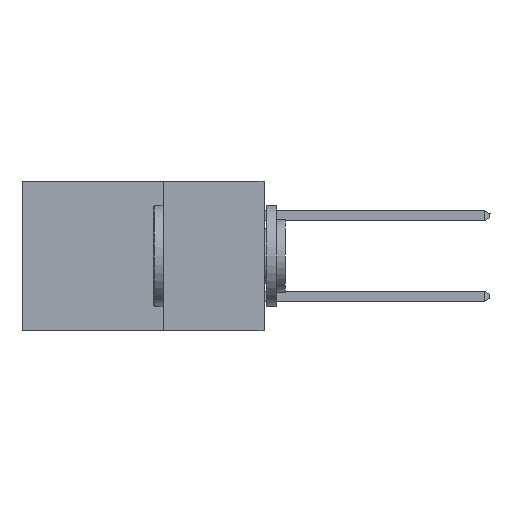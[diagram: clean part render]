
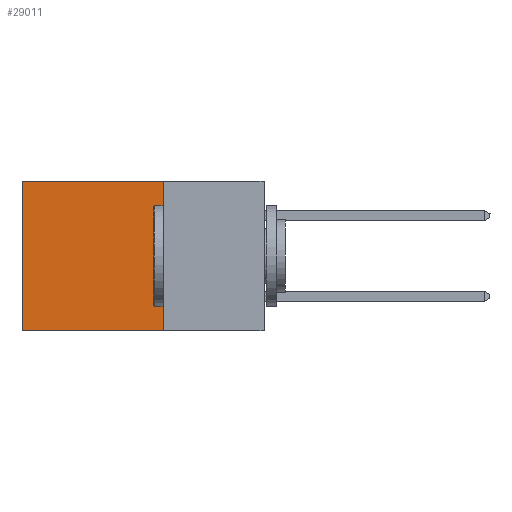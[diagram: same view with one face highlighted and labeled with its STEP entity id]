
A CAD part, left-side view. The second image highlights one B-rep face of the part: STEP entity #29011.
In plain terms, the highlighted planar face has unit normal (-1, 0, 0).
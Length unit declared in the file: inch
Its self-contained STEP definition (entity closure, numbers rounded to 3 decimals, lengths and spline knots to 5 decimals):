
#53 = EDGE_CURVE ( 'NONE', #11010, #13766, #13599, .T. ) ;
#420 = ORIENTED_EDGE ( 'NONE', *, *, #2984, .F. ) ;
#733 = CARTESIAN_POINT ( 'NONE',  ( 0.298, 0.6, 0. ) ) ;
#2420 = ORIENTED_EDGE ( 'NONE', *, *, #22409, .F. ) ;
#2984 = EDGE_CURVE ( 'NONE', #11010, #21781, #19633, .T. ) ;
#4098 = VECTOR ( 'NONE', #16727, 39.37008 ) ;
#4325 = DIRECTION ( 'NONE',  ( 0., 1., 0. ) ) ;
#5037 = EDGE_LOOP ( 'NONE', ( #10179, #2420, #420, #7628 ) ) ;
#7579 = LINE ( 'NONE', #29816, #13073 ) ;
#7628 = ORIENTED_EDGE ( 'NONE', *, *, #53, .T. ) ;
#10179 = ORIENTED_EDGE ( 'NONE', *, *, #11379, .T. ) ;
#10982 = PLANE ( 'NONE',  #29742 ) ;
#11010 = VERTEX_POINT ( 'NONE', #24628 ) ;
#11379 = EDGE_CURVE ( 'NONE', #13766, #21625, #23343, .T. ) ;
#12746 = CARTESIAN_POINT ( 'NONE',  ( 0.298, 0.25, 0. ) ) ;
#13073 = VECTOR ( 'NONE', #4325, 39.37008 ) ;
#13345 = CARTESIAN_POINT ( 'NONE',  ( 0.298, 0.25, 0. ) ) ;
#13599 = LINE ( 'NONE', #22478, #20125 ) ;
#13766 = VERTEX_POINT ( 'NONE', #22774 ) ;
#16727 = DIRECTION ( 'NONE',  ( 0., 0., -1. ) ) ;
#17180 = DIRECTION ( 'NONE',  ( 0., 0., -1. ) ) ;
#17198 = CARTESIAN_POINT ( 'NONE',  ( 0.298, 0.6, -0.37 ) ) ;
#17972 = DIRECTION ( 'NONE',  ( 1., 0., 0. ) ) ;
#18889 = VECTOR ( 'NONE', #17180, 39.37008 ) ;
#19633 = LINE ( 'NONE', #12746, #18889 ) ;
#20125 = VECTOR ( 'NONE', #24868, 39.37008 ) ;
#21625 = VERTEX_POINT ( 'NONE', #17198 ) ;
#21781 = VERTEX_POINT ( 'NONE', #27201 ) ;
#22409 = EDGE_CURVE ( 'NONE', #21781, #21625, #7579, .T. ) ;
#22478 = CARTESIAN_POINT ( 'NONE',  ( 0.298, 0.25, 0. ) ) ;
#22634 = DIRECTION ( 'NONE',  ( 0., 0., -1. ) ) ;
#22774 = CARTESIAN_POINT ( 'NONE',  ( 0.298, 0.6, 0. ) ) ;
#23343 = LINE ( 'NONE', #733, #4098 ) ;
#23355 = FACE_OUTER_BOUND ( 'NONE', #5037, .T. ) ;
#24628 = CARTESIAN_POINT ( 'NONE',  ( 0.298, 0.25, 0. ) ) ;
#24868 = DIRECTION ( 'NONE',  ( 0., 1., 0. ) ) ;
#27201 = CARTESIAN_POINT ( 'NONE',  ( 0.298, 0.25, -0.37 ) ) ;
#29011 = ADVANCED_FACE ( 'NONE', ( #23355 ), #10982, .F. ) ;
#29742 = AXIS2_PLACEMENT_3D ( 'NONE', #13345, #17972, #22634 ) ;
#29816 = CARTESIAN_POINT ( 'NONE',  ( 0.298, 0.25, -0.37 ) ) ;
